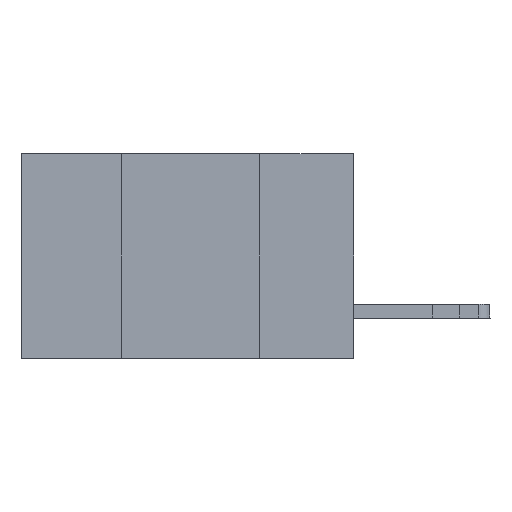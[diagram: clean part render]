
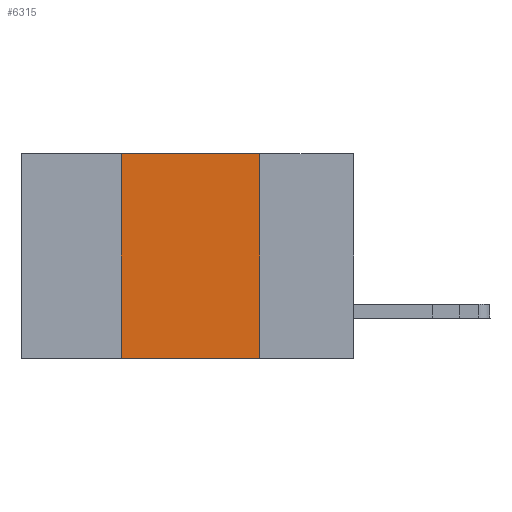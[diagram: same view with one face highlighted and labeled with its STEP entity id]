
A CAD part, left-side view. The second image highlights one B-rep face of the part: STEP entity #6315.
In plain terms, the highlighted planar face has unit normal (-1, 0, 0).
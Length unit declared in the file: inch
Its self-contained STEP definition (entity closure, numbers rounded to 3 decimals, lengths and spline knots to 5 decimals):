
#52 = VECTOR ( 'NONE', #20253, 39.37008 ) ;
#149 = VECTOR ( 'NONE', #21878, 39.37008 ) ;
#152 = LINE ( 'NONE', #11417, #10444 ) ;
#371 = ORIENTED_EDGE ( 'NONE', *, *, #24470, .T. ) ;
#1007 = LINE ( 'NONE', #1237, #52 ) ;
#1067 = EDGE_CURVE ( 'NONE', #3180, #18383, #23522, .T. ) ;
#1237 = CARTESIAN_POINT ( 'NONE',  ( 0., 0.17, 0. ) ) ;
#2102 = DIRECTION ( 'NONE',  ( 0., 0., -1. ) ) ;
#2979 = EDGE_LOOP ( 'NONE', ( #14750, #10653, #11270, #371 ) ) ;
#3163 = EDGE_CURVE ( 'NONE', #18383, #7331, #1007, .T. ) ;
#3180 = VERTEX_POINT ( 'NONE', #25444 ) ;
#5887 = FACE_OUTER_BOUND ( 'NONE', #2979, .T. ) ;
#6315 = ADVANCED_FACE ( 'NONE', ( #5887 ), #26124, .F. ) ;
#6984 = VECTOR ( 'NONE', #16249, 39.37008 ) ;
#7072 = CARTESIAN_POINT ( 'NONE',  ( 0., 0.17, 0. ) ) ;
#7331 = VERTEX_POINT ( 'NONE', #13488 ) ;
#7478 = CARTESIAN_POINT ( 'NONE',  ( 0., 0.6, 0. ) ) ;
#10203 = CARTESIAN_POINT ( 'NONE',  ( 0., 0.6, 0. ) ) ;
#10444 = VECTOR ( 'NONE', #13437, 39.37008 ) ;
#10653 = ORIENTED_EDGE ( 'NONE', *, *, #1067, .F. ) ;
#11270 = ORIENTED_EDGE ( 'NONE', *, *, #15440, .F. ) ;
#11417 = CARTESIAN_POINT ( 'NONE',  ( 0., 0.42, 0. ) ) ;
#11895 = CARTESIAN_POINT ( 'NONE',  ( 0., 0.6, -0.37 ) ) ;
#11910 = CARTESIAN_POINT ( 'NONE',  ( 0., 0.42, -0.37 ) ) ;
#13437 = DIRECTION ( 'NONE',  ( 0., 0., 1. ) ) ;
#13488 = CARTESIAN_POINT ( 'NONE',  ( 0., 0.17, -0.37 ) ) ;
#14241 = DIRECTION ( 'NONE',  ( 1., 0., 0. ) ) ;
#14750 = ORIENTED_EDGE ( 'NONE', *, *, #3163, .F. ) ;
#15440 = EDGE_CURVE ( 'NONE', #16877, #3180, #152, .T. ) ;
#15758 = AXIS2_PLACEMENT_3D ( 'NONE', #10203, #14241, #2102 ) ;
#16249 = DIRECTION ( 'NONE',  ( 0., -1., 0. ) ) ;
#16877 = VERTEX_POINT ( 'NONE', #11910 ) ;
#18383 = VERTEX_POINT ( 'NONE', #7072 ) ;
#20253 = DIRECTION ( 'NONE',  ( 0., 0., -1. ) ) ;
#21705 = LINE ( 'NONE', #11895, #149 ) ;
#21878 = DIRECTION ( 'NONE',  ( 0., -1., 0. ) ) ;
#23522 = LINE ( 'NONE', #7478, #6984 ) ;
#24470 = EDGE_CURVE ( 'NONE', #16877, #7331, #21705, .T. ) ;
#25444 = CARTESIAN_POINT ( 'NONE',  ( 0., 0.42, 0. ) ) ;
#26124 = PLANE ( 'NONE',  #15758 ) ;
